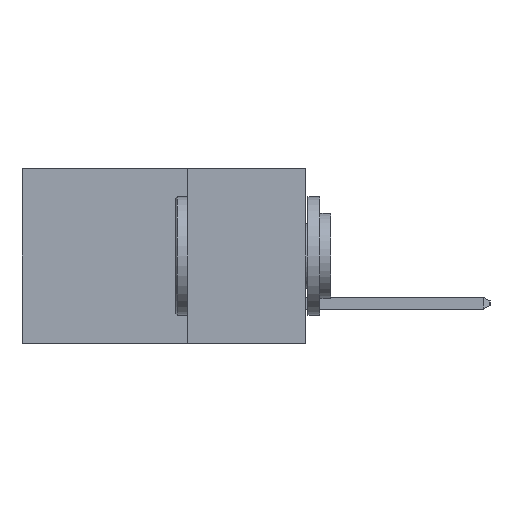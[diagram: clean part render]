
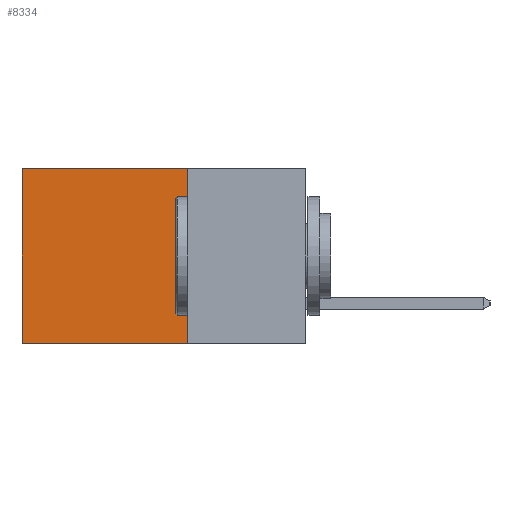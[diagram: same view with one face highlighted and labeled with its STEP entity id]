
A CAD part, left-side view. The second image highlights one B-rep face of the part: STEP entity #8334.
In plain terms, the highlighted planar face has unit normal (-1, 0, 0).
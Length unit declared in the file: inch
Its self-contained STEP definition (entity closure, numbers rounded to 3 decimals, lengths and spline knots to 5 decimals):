
#73 = EDGE_CURVE ( 'NONE', #1849, #4165, #10060, .T. ) ;
#134 = DIRECTION ( 'NONE',  ( 0., 0., -1. ) ) ;
#292 = AXIS2_PLACEMENT_3D ( 'NONE', #5235, #3338, #10054 ) ;
#516 = LINE ( 'NONE', #9198, #7994 ) ;
#820 = CARTESIAN_POINT ( 'NONE',  ( 0.298, 0.6, 0. ) ) ;
#1849 = VERTEX_POINT ( 'NONE', #7490 ) ;
#2114 = EDGE_LOOP ( 'NONE', ( #5939, #6092, #11321, #2508 ) ) ;
#2368 = PLANE ( 'NONE',  #292 ) ;
#2508 = ORIENTED_EDGE ( 'NONE', *, *, #5866, .T. ) ;
#3118 = VECTOR ( 'NONE', #4813, 39.37008 ) ;
#3338 = DIRECTION ( 'NONE',  ( 1., 0., 0. ) ) ;
#3586 = CARTESIAN_POINT ( 'NONE',  ( 0.298, 0.25, -0.37 ) ) ;
#3610 = CARTESIAN_POINT ( 'NONE',  ( 0.298, 0.25, 0. ) ) ;
#3728 = DIRECTION ( 'NONE',  ( 0., 1., 0. ) ) ;
#4165 = VERTEX_POINT ( 'NONE', #12062 ) ;
#4769 = CARTESIAN_POINT ( 'NONE',  ( 0.298, 0.25, 0. ) ) ;
#4813 = DIRECTION ( 'NONE',  ( 0., 1., 0. ) ) ;
#4923 = VERTEX_POINT ( 'NONE', #820 ) ;
#5235 = CARTESIAN_POINT ( 'NONE',  ( 0.298, 0.25, 0. ) ) ;
#5712 = LINE ( 'NONE', #4769, #3118 ) ;
#5866 = EDGE_CURVE ( 'NONE', #6581, #4923, #5712, .T. ) ;
#5883 = EDGE_CURVE ( 'NONE', #4923, #4165, #516, .T. ) ;
#5939 = ORIENTED_EDGE ( 'NONE', *, *, #5883, .T. ) ;
#6092 = ORIENTED_EDGE ( 'NONE', *, *, #73, .F. ) ;
#6581 = VERTEX_POINT ( 'NONE', #3610 ) ;
#7278 = VECTOR ( 'NONE', #3728, 39.37008 ) ;
#7490 = CARTESIAN_POINT ( 'NONE',  ( 0.298, 0.25, -0.37 ) ) ;
#7994 = VECTOR ( 'NONE', #8763, 39.37008 ) ;
#8334 = ADVANCED_FACE ( 'NONE', ( #10489 ), #2368, .F. ) ;
#8763 = DIRECTION ( 'NONE',  ( 0., 0., -1. ) ) ;
#8803 = EDGE_CURVE ( 'NONE', #6581, #1849, #12257, .T. ) ;
#9198 = CARTESIAN_POINT ( 'NONE',  ( 0.298, 0.6, 0. ) ) ;
#10054 = DIRECTION ( 'NONE',  ( 0., 0., -1. ) ) ;
#10060 = LINE ( 'NONE', #3586, #7278 ) ;
#10489 = FACE_OUTER_BOUND ( 'NONE', #2114, .T. ) ;
#11321 = ORIENTED_EDGE ( 'NONE', *, *, #8803, .F. ) ;
#11515 = CARTESIAN_POINT ( 'NONE',  ( 0.298, 0.25, 0. ) ) ;
#11972 = VECTOR ( 'NONE', #134, 39.37008 ) ;
#12062 = CARTESIAN_POINT ( 'NONE',  ( 0.298, 0.6, -0.37 ) ) ;
#12257 = LINE ( 'NONE', #11515, #11972 ) ;
